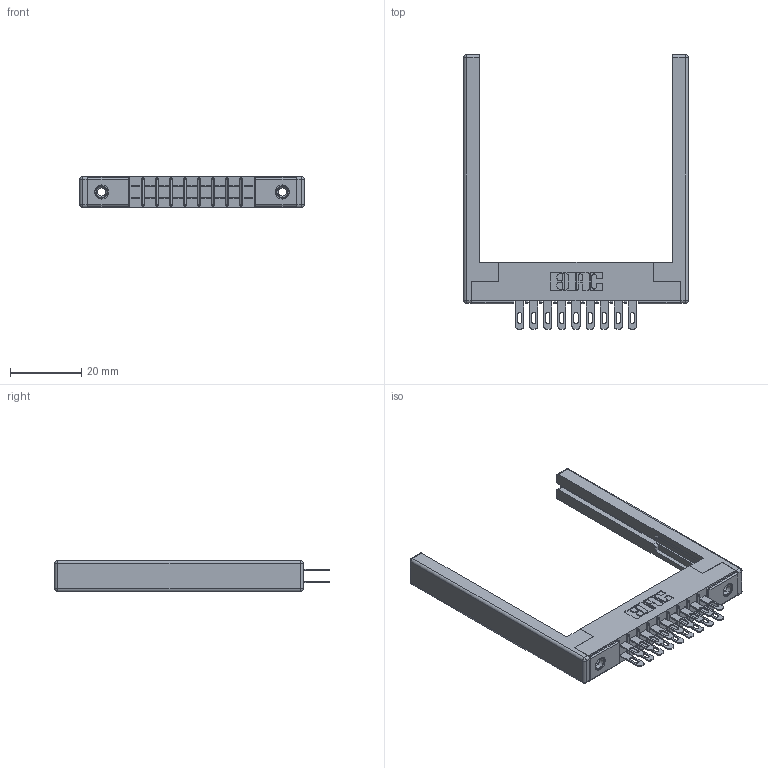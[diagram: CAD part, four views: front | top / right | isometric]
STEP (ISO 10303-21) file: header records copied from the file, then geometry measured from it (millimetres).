
FILE_DESCRIPTION (( 'STEP AP203' ), '1' );
FILE_NAME ('355-018-500-268.STEP', '2019-09-11T02:27:00', ( '' ), ( '' ), 'SwSTEP 2.0', 'SolidWorks 2016', '' );
FILE_SCHEMA (( 'CONFIG_CONTROL_DESIGN' ));
Length unit declared in the file: inch
Products named in the file (5): 355-018-500-268; 307-220-068; 345-250-001_345-250-001-102; 305-290-001_500; 305 Part_.156 Dia
Assembly tree (23 placements, depth 2):
  355-018-500-268
    305 Part_.156 Dia
    305-290-001_500  x18
    345-250-001_345-250-001-102  x2
    307-220-068  x2
Bounding box: 63.09 x 77.14 x 8.71 mm (x, y, z)
Volume: 8601.8 mm3; surface area: 11202.2 mm2
Topology: 23 solids, 23 shells, 1170 faces, 3289 edges, 2122 vertices
Faces by surface type: plane 660, cylinder 450, sphere 44, cone 12, torus 4
Entity records: 16543 total; most frequent: CARTESIAN_POINT 2710, ORIENTED_EDGE 2676, DIRECTION 2670, EDGE_CURVE 1338, LINE 1034, VECTOR 1034, VERTEX_POINT 858, AXIS2_PLACEMENT_3D 818
